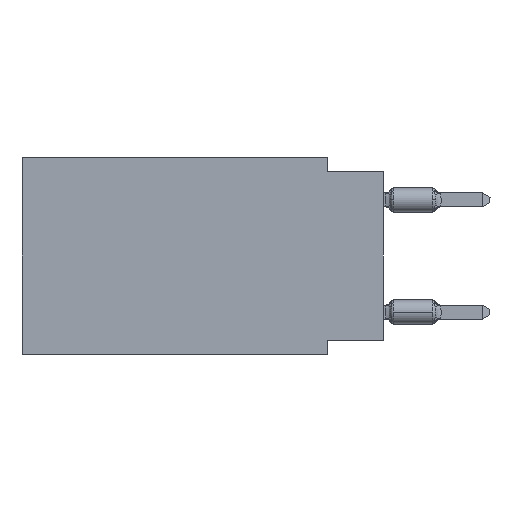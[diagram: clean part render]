
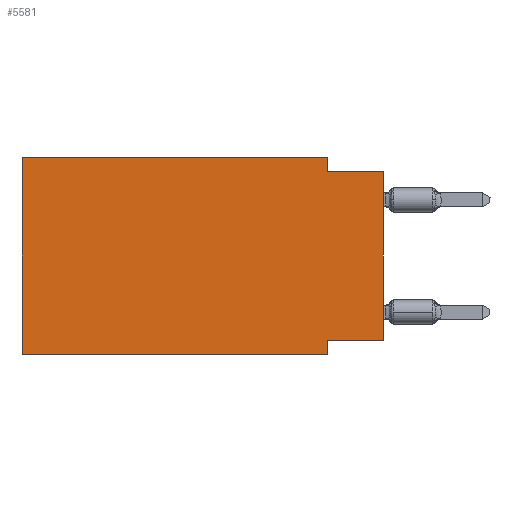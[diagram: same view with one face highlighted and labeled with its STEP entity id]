
A CAD part, left-side view. The second image highlights one B-rep face of the part: STEP entity #5581.
In plain terms, the highlighted planar face has unit normal (-1, 0, 0).
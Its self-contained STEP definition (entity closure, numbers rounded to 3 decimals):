
#398 = CARTESIAN_POINT ( 'NONE',  ( 0., 2.54, -8.255 ) ) ;
#1069 = AXIS2_PLACEMENT_3D ( 'NONE', #3203, #10642, #19314 ) ;
#1574 = VERTEX_POINT ( 'NONE', #32600 ) ;
#2666 = EDGE_CURVE ( 'NONE', #29100, #37205, #7550, .T. ) ;
#3203 = CARTESIAN_POINT ( 'NONE',  ( 0., 16.383, 0. ) ) ;
#3844 = CARTESIAN_POINT ( 'NONE',  ( 0., 0., -8.255 ) ) ;
#4740 = EDGE_CURVE ( 'NONE', #37016, #37205, #28990, .T. ) ;
#4958 = ORIENTED_EDGE ( 'NONE', *, *, #6752, .F. ) ;
#5190 = VERTEX_POINT ( 'NONE', #15785 ) ;
#5581 = ADVANCED_FACE ( 'NONE', ( #37993 ), #46699, .F. ) ;
#5755 = EDGE_CURVE ( 'NONE', #1574, #5190, #24425, .T. ) ;
#6019 = CARTESIAN_POINT ( 'NONE',  ( 0., 2.54, 0. ) ) ;
#6722 = EDGE_CURVE ( 'NONE', #37016, #7412, #28646, .T. ) ;
#6752 = EDGE_CURVE ( 'NONE', #7412, #46071, #25316, .T. ) ;
#7412 = VERTEX_POINT ( 'NONE', #43560 ) ;
#7550 = LINE ( 'NONE', #11636, #39099 ) ;
#7629 = EDGE_LOOP ( 'NONE', ( #22632, #41346, #33384, #4958, #16512, #33328, #42532, #30406 ) ) ;
#8663 = LINE ( 'NONE', #24266, #10976 ) ;
#9826 = DIRECTION ( 'NONE',  ( 0., -1., 0. ) ) ;
#10470 = VECTOR ( 'NONE', #27135, 1000. ) ;
#10642 = DIRECTION ( 'NONE',  ( 1., 0., 0. ) ) ;
#10870 = DIRECTION ( 'NONE',  ( 0., 0., -1. ) ) ;
#10976 = VECTOR ( 'NONE', #39873, 1000. ) ;
#11636 = CARTESIAN_POINT ( 'NONE',  ( 0., 2.54, -8.89 ) ) ;
#13920 = EDGE_CURVE ( 'NONE', #46071, #41156, #41317, .T. ) ;
#15785 = CARTESIAN_POINT ( 'NONE',  ( 0., 0., -0.635 ) ) ;
#16512 = ORIENTED_EDGE ( 'NONE', *, *, #6722, .F. ) ;
#16612 = DIRECTION ( 'NONE',  ( 0., 0., 1. ) ) ;
#17276 = CARTESIAN_POINT ( 'NONE',  ( 0., 16.383, -8.89 ) ) ;
#17617 = DIRECTION ( 'NONE',  ( 0., -1., 0. ) ) ;
#17688 = CARTESIAN_POINT ( 'NONE',  ( 0., 2.54, -0.635 ) ) ;
#19314 = DIRECTION ( 'NONE',  ( 0., 0., -1. ) ) ;
#22145 = VECTOR ( 'NONE', #10870, 1000. ) ;
#22632 = ORIENTED_EDGE ( 'NONE', *, *, #5755, .T. ) ;
#24266 = CARTESIAN_POINT ( 'NONE',  ( 0., 0., -0.635 ) ) ;
#24425 = LINE ( 'NONE', #27995, #50131 ) ;
#24563 = CARTESIAN_POINT ( 'NONE',  ( 0., 16.383, 0. ) ) ;
#25316 = LINE ( 'NONE', #25548, #27724 ) ;
#25548 = CARTESIAN_POINT ( 'NONE',  ( 0., 16.383, 0. ) ) ;
#25752 = CARTESIAN_POINT ( 'NONE',  ( 0., 2.54, 0. ) ) ;
#27135 = DIRECTION ( 'NONE',  ( 0., 1., 0. ) ) ;
#27724 = VECTOR ( 'NONE', #17617, 1000. ) ;
#27995 = CARTESIAN_POINT ( 'NONE',  ( 0., 0., 0. ) ) ;
#28646 = LINE ( 'NONE', #24563, #43236 ) ;
#28990 = LINE ( 'NONE', #41251, #43457 ) ;
#29100 = VERTEX_POINT ( 'NONE', #398 ) ;
#30406 = ORIENTED_EDGE ( 'NONE', *, *, #36532, .F. ) ;
#32424 = EDGE_CURVE ( 'NONE', #41156, #5190, #8663, .T. ) ;
#32600 = CARTESIAN_POINT ( 'NONE',  ( 0., 0., -8.255 ) ) ;
#33328 = ORIENTED_EDGE ( 'NONE', *, *, #4740, .T. ) ;
#33384 = ORIENTED_EDGE ( 'NONE', *, *, #13920, .F. ) ;
#35419 = DIRECTION ( 'NONE',  ( 0., 0., -1. ) ) ;
#36532 = EDGE_CURVE ( 'NONE', #1574, #29100, #38637, .T. ) ;
#37016 = VERTEX_POINT ( 'NONE', #17276 ) ;
#37205 = VERTEX_POINT ( 'NONE', #49235 ) ;
#37993 = FACE_OUTER_BOUND ( 'NONE', #7629, .T. ) ;
#38637 = LINE ( 'NONE', #3844, #10470 ) ;
#39099 = VECTOR ( 'NONE', #35419, 1000. ) ;
#39269 = DIRECTION ( 'NONE',  ( 0., 0., 1. ) ) ;
#39873 = DIRECTION ( 'NONE',  ( 0., -1., 0. ) ) ;
#41156 = VERTEX_POINT ( 'NONE', #17688 ) ;
#41251 = CARTESIAN_POINT ( 'NONE',  ( 0., 16.383, -8.89 ) ) ;
#41317 = LINE ( 'NONE', #6019, #22145 ) ;
#41346 = ORIENTED_EDGE ( 'NONE', *, *, #32424, .F. ) ;
#42532 = ORIENTED_EDGE ( 'NONE', *, *, #2666, .F. ) ;
#43236 = VECTOR ( 'NONE', #16612, 1000. ) ;
#43457 = VECTOR ( 'NONE', #9826, 1000. ) ;
#43560 = CARTESIAN_POINT ( 'NONE',  ( 0., 16.383, 0. ) ) ;
#46071 = VERTEX_POINT ( 'NONE', #25752 ) ;
#46699 = PLANE ( 'NONE',  #1069 ) ;
#49235 = CARTESIAN_POINT ( 'NONE',  ( 0., 2.54, -8.89 ) ) ;
#50131 = VECTOR ( 'NONE', #39269, 1000. ) ;
